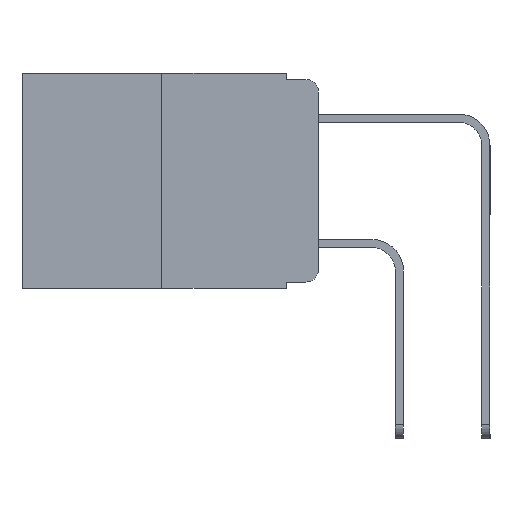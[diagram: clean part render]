
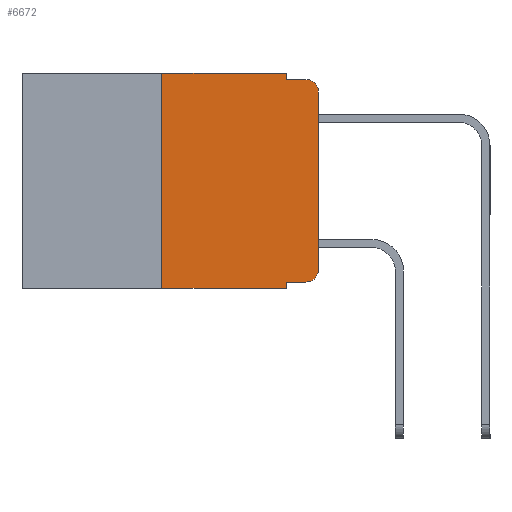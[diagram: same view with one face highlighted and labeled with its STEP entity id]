
A CAD part, left-side view. The second image highlights one B-rep face of the part: STEP entity #6672.
In plain terms, the highlighted planar face has unit normal (-1, 0, 0).
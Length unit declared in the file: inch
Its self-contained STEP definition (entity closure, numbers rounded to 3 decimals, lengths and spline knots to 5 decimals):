
#336 = VECTOR ( 'NONE', #20237, 39.37008 ) ;
#435 = ORIENTED_EDGE ( 'NONE', *, *, #14787, .F. ) ;
#464 = CARTESIAN_POINT ( 'NONE',  ( 0., 0.051, -0.343 ) ) ;
#747 = ORIENTED_EDGE ( 'NONE', *, *, #20534, .T. ) ;
#1249 = VERTEX_POINT ( 'NONE', #22422 ) ;
#1336 = ORIENTED_EDGE ( 'NONE', *, *, #7851, .T. ) ;
#1614 = CARTESIAN_POINT ( 'NONE',  ( 0., 0.02, -0.313 ) ) ;
#1734 = VERTEX_POINT ( 'NONE', #5494 ) ;
#2314 = AXIS2_PLACEMENT_3D ( 'NONE', #13153, #2440, #14832 ) ;
#2346 = VECTOR ( 'NONE', #21265, 39.37008 ) ;
#2401 = DIRECTION ( 'NONE',  ( 0., 0., -1. ) ) ;
#2440 = DIRECTION ( 'NONE',  ( -1., 0., 0. ) ) ;
#2605 = VERTEX_POINT ( 'NONE', #15070 ) ;
#2709 = LINE ( 'NONE', #13473, #20787 ) ;
#2810 = CARTESIAN_POINT ( 'NONE',  ( 0., 0.051, -0.01 ) ) ;
#2869 = DIRECTION ( 'NONE',  ( 0., 0., 1. ) ) ;
#3178 = LINE ( 'NONE', #21313, #16621 ) ;
#3508 = DIRECTION ( 'NONE',  ( 0., 0., -1. ) ) ;
#3927 = VERTEX_POINT ( 'NONE', #20044 ) ;
#4240 = VERTEX_POINT ( 'NONE', #13988 ) ;
#4317 = CARTESIAN_POINT ( 'NONE',  ( 0., 0.25, 0. ) ) ;
#5494 = CARTESIAN_POINT ( 'NONE',  ( 0., 0.051, -0.01 ) ) ;
#5699 = CARTESIAN_POINT ( 'NONE',  ( 0., 0.051, -0.333 ) ) ;
#5819 = FACE_OUTER_BOUND ( 'NONE', #20505, .T. ) ;
#5929 = VERTEX_POINT ( 'NONE', #7662 ) ;
#5936 = CIRCLE ( 'NONE', #2314, 0.02 ) ;
#6423 = CARTESIAN_POINT ( 'NONE',  ( 0., 0.051, 0. ) ) ;
#6608 = VERTEX_POINT ( 'NONE', #17964 ) ;
#6672 = ADVANCED_FACE ( 'NONE', ( #5819 ), #19881, .F. ) ;
#6818 = DIRECTION ( 'NONE',  ( 0., -1., 0. ) ) ;
#6950 = EDGE_CURVE ( 'NONE', #3927, #11850, #13237, .T. ) ;
#6954 = VECTOR ( 'NONE', #7878, 39.37008 ) ;
#7246 = LINE ( 'NONE', #5699, #2346 ) ;
#7409 = LINE ( 'NONE', #2810, #20069 ) ;
#7444 = ORIENTED_EDGE ( 'NONE', *, *, #18177, .F. ) ;
#7534 = LINE ( 'NONE', #13067, #6954 ) ;
#7662 = CARTESIAN_POINT ( 'NONE',  ( 0., 0.02, -0.01 ) ) ;
#7851 = EDGE_CURVE ( 'NONE', #4240, #2605, #21290, .T. ) ;
#7878 = DIRECTION ( 'NONE',  ( 0., 0., -1. ) ) ;
#8392 = DIRECTION ( 'NONE',  ( 0., 0., 1. ) ) ;
#8515 = VERTEX_POINT ( 'NONE', #6423 ) ;
#8602 = VECTOR ( 'NONE', #6818, 39.37008 ) ;
#9050 = EDGE_CURVE ( 'NONE', #6608, #4240, #7246, .T. ) ;
#9163 = AXIS2_PLACEMENT_3D ( 'NONE', #1614, #14121, #3508 ) ;
#9658 = EDGE_CURVE ( 'NONE', #19394, #8515, #3178, .T. ) ;
#10001 = CARTESIAN_POINT ( 'NONE',  ( 0., 0.051, 0. ) ) ;
#10743 = ORIENTED_EDGE ( 'NONE', *, *, #6950, .T. ) ;
#11008 = ORIENTED_EDGE ( 'NONE', *, *, #9658, .F. ) ;
#11850 = VERTEX_POINT ( 'NONE', #464 ) ;
#12735 = VECTOR ( 'NONE', #2869, 39.37008 ) ;
#12822 = DIRECTION ( 'NONE',  ( 0., -1., 0. ) ) ;
#13067 = CARTESIAN_POINT ( 'NONE',  ( 0., 0.051, 0. ) ) ;
#13122 = DIRECTION ( 'NONE',  ( 1., 0., 0. ) ) ;
#13153 = CARTESIAN_POINT ( 'NONE',  ( 0., 0.02, -0.03 ) ) ;
#13237 = LINE ( 'NONE', #17125, #8602 ) ;
#13473 = CARTESIAN_POINT ( 'NONE',  ( 0., 0., 0. ) ) ;
#13671 = EDGE_CURVE ( 'NONE', #6608, #11850, #19166, .T. ) ;
#13988 = CARTESIAN_POINT ( 'NONE',  ( 0., 0.02, -0.333 ) ) ;
#14121 = DIRECTION ( 'NONE',  ( -1., 0., 0. ) ) ;
#14787 = EDGE_CURVE ( 'NONE', #3927, #19394, #17196, .T. ) ;
#14832 = DIRECTION ( 'NONE',  ( 0., 0., -1. ) ) ;
#15070 = CARTESIAN_POINT ( 'NONE',  ( 0., 0., -0.313 ) ) ;
#15764 = ORIENTED_EDGE ( 'NONE', *, *, #13671, .F. ) ;
#15902 = EDGE_CURVE ( 'NONE', #8515, #1734, #7534, .T. ) ;
#16621 = VECTOR ( 'NONE', #12822, 39.37008 ) ;
#17092 = ORIENTED_EDGE ( 'NONE', *, *, #15902, .F. ) ;
#17125 = CARTESIAN_POINT ( 'NONE',  ( 0., 0.473, -0.343 ) ) ;
#17196 = LINE ( 'NONE', #20329, #12735 ) ;
#17964 = CARTESIAN_POINT ( 'NONE',  ( 0., 0.051, -0.333 ) ) ;
#18111 = CARTESIAN_POINT ( 'NONE',  ( 0., 0.473, 0. ) ) ;
#18177 = EDGE_CURVE ( 'NONE', #1734, #5929, #7409, .T. ) ;
#18860 = AXIS2_PLACEMENT_3D ( 'NONE', #18111, #13122, #2401 ) ;
#19166 = LINE ( 'NONE', #10001, #336 ) ;
#19370 = EDGE_CURVE ( 'NONE', #1249, #5929, #5936, .T. ) ;
#19394 = VERTEX_POINT ( 'NONE', #4317 ) ;
#19547 = ORIENTED_EDGE ( 'NONE', *, *, #9050, .T. ) ;
#19881 = PLANE ( 'NONE',  #18860 ) ;
#20044 = CARTESIAN_POINT ( 'NONE',  ( 0., 0.25, -0.343 ) ) ;
#20069 = VECTOR ( 'NONE', #22052, 39.37008 ) ;
#20237 = DIRECTION ( 'NONE',  ( 0., 0., -1. ) ) ;
#20329 = CARTESIAN_POINT ( 'NONE',  ( 0., 0.25, 0. ) ) ;
#20505 = EDGE_LOOP ( 'NONE', ( #747, #20629, #7444, #17092, #11008, #435, #10743, #15764, #19547, #1336 ) ) ;
#20534 = EDGE_CURVE ( 'NONE', #2605, #1249, #2709, .T. ) ;
#20629 = ORIENTED_EDGE ( 'NONE', *, *, #19370, .T. ) ;
#20787 = VECTOR ( 'NONE', #8392, 39.37008 ) ;
#21265 = DIRECTION ( 'NONE',  ( 0., -1., 0. ) ) ;
#21290 = CIRCLE ( 'NONE', #9163, 0.02 ) ;
#21313 = CARTESIAN_POINT ( 'NONE',  ( 0., 0.473, 0. ) ) ;
#22052 = DIRECTION ( 'NONE',  ( 0., -1., 0. ) ) ;
#22422 = CARTESIAN_POINT ( 'NONE',  ( 0., 0., -0.03 ) ) ;
